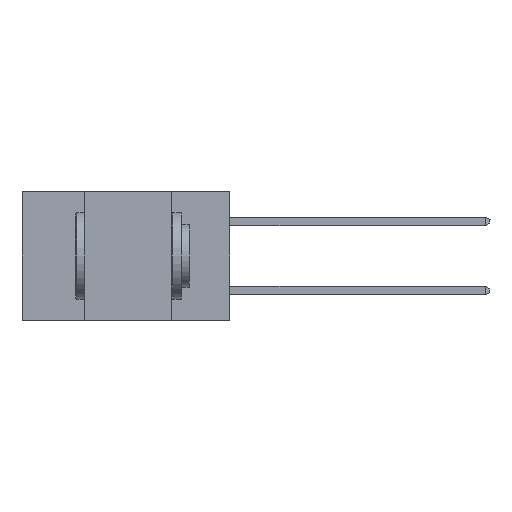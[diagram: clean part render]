
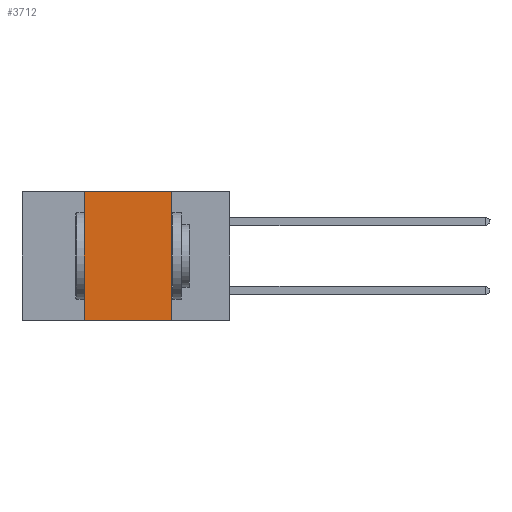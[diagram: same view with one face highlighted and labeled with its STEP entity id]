
A CAD part, left-side view. The second image highlights one B-rep face of the part: STEP entity #3712.
In plain terms, the highlighted planar face has unit normal (-1, 0, 0).
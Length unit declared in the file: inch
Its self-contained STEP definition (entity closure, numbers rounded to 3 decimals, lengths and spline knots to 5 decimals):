
#595 = LINE ( 'NONE', #7389, #8885 ) ;
#1456 = VECTOR ( 'NONE', #9211, 39.37008 ) ;
#2046 = EDGE_LOOP ( 'NONE', ( #3964, #6428, #8803, #7113 ) ) ;
#2169 = DIRECTION ( 'NONE',  ( 1., 0., 0. ) ) ;
#2316 = CARTESIAN_POINT ( 'NONE',  ( 0., 0.17, -0.37 ) ) ;
#2707 = LINE ( 'NONE', #20991, #11515 ) ;
#3359 = AXIS2_PLACEMENT_3D ( 'NONE', #18737, #2169, #20872 ) ;
#3712 = ADVANCED_FACE ( 'NONE', ( #3832 ), #13523, .F. ) ;
#3832 = FACE_OUTER_BOUND ( 'NONE', #2046, .T. ) ;
#3964 = ORIENTED_EDGE ( 'NONE', *, *, #15260, .F. ) ;
#4034 = VERTEX_POINT ( 'NONE', #19825 ) ;
#6428 = ORIENTED_EDGE ( 'NONE', *, *, #13717, .F. ) ;
#6807 = LINE ( 'NONE', #18705, #11328 ) ;
#7113 = ORIENTED_EDGE ( 'NONE', *, *, #21430, .T. ) ;
#7389 = CARTESIAN_POINT ( 'NONE',  ( 0., 0.6, 0. ) ) ;
#8044 = CARTESIAN_POINT ( 'NONE',  ( 0., 0.17, 0. ) ) ;
#8803 = ORIENTED_EDGE ( 'NONE', *, *, #12612, .F. ) ;
#8885 = VECTOR ( 'NONE', #15955, 39.37008 ) ;
#9211 = DIRECTION ( 'NONE',  ( 0., 0., -1. ) ) ;
#9496 = DIRECTION ( 'NONE',  ( 0., -1., 0. ) ) ;
#10652 = VERTEX_POINT ( 'NONE', #13864 ) ;
#10805 = VERTEX_POINT ( 'NONE', #8044 ) ;
#11089 = LINE ( 'NONE', #2316, #1456 ) ;
#11328 = VECTOR ( 'NONE', #13591, 39.37008 ) ;
#11515 = VECTOR ( 'NONE', #9496, 39.37008 ) ;
#12612 = EDGE_CURVE ( 'NONE', #4034, #10652, #6807, .T. ) ;
#13242 = CARTESIAN_POINT ( 'NONE',  ( 0., 0.17, -0.37 ) ) ;
#13523 = PLANE ( 'NONE',  #3359 ) ;
#13591 = DIRECTION ( 'NONE',  ( 0., 0., 1. ) ) ;
#13717 = EDGE_CURVE ( 'NONE', #10652, #10805, #595, .T. ) ;
#13864 = CARTESIAN_POINT ( 'NONE',  ( 0., 0.42, 0. ) ) ;
#14490 = VERTEX_POINT ( 'NONE', #13242 ) ;
#15260 = EDGE_CURVE ( 'NONE', #10805, #14490, #11089, .T. ) ;
#15955 = DIRECTION ( 'NONE',  ( 0., -1., 0. ) ) ;
#18705 = CARTESIAN_POINT ( 'NONE',  ( 0., 0.42, -0.37 ) ) ;
#18737 = CARTESIAN_POINT ( 'NONE',  ( 0., 0.6, 0. ) ) ;
#19825 = CARTESIAN_POINT ( 'NONE',  ( 0., 0.42, -0.37 ) ) ;
#20872 = DIRECTION ( 'NONE',  ( 0., 0., -1. ) ) ;
#20991 = CARTESIAN_POINT ( 'NONE',  ( 0., 0.6, -0.37 ) ) ;
#21430 = EDGE_CURVE ( 'NONE', #4034, #14490, #2707, .T. ) ;
